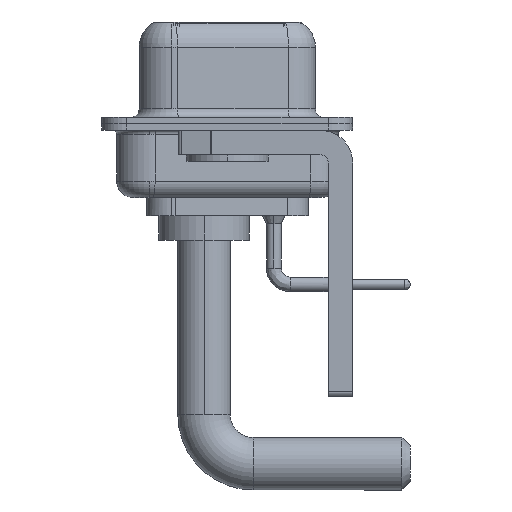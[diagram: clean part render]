
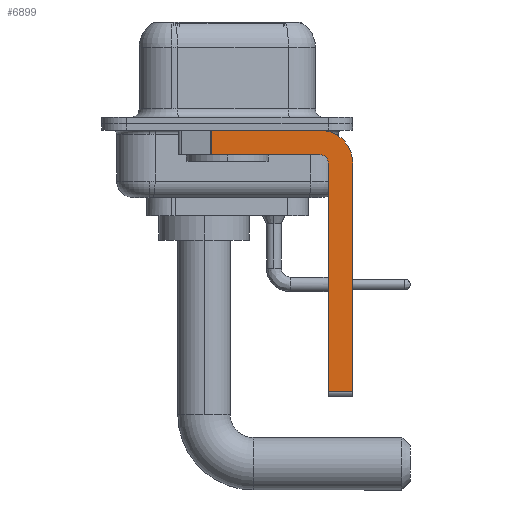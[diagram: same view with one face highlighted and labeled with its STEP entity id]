
A CAD part, left-side view. The second image highlights one B-rep face of the part: STEP entity #6899.
In plain terms, the highlighted planar face has unit normal (-1, 0, 0).
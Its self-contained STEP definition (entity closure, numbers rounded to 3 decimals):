
#76 = VERTEX_POINT ( 'NONE', #11572 ) ;
#138 = AXIS2_PLACEMENT_3D ( 'NONE', #9289, #16056, #19088 ) ;
#366 = CARTESIAN_POINT ( 'NONE',  ( -2.9, -5.65, -0.4 ) ) ;
#731 = LINE ( 'NONE', #9382, #17264 ) ;
#1268 = PLANE ( 'NONE',  #7855 ) ;
#1321 = EDGE_CURVE ( 'NONE', #5923, #15533, #731, .T. ) ;
#2050 = LINE ( 'NONE', #2499, #5967 ) ;
#2391 = ORIENTED_EDGE ( 'NONE', *, *, #16964, .T. ) ;
#2499 = CARTESIAN_POINT ( 'NONE',  ( -2.9, -6.15, -16.6 ) ) ;
#3042 = EDGE_CURVE ( 'NONE', #18371, #21373, #4157, .T. ) ;
#4157 = LINE ( 'NONE', #4265, #19588 ) ;
#4265 = CARTESIAN_POINT ( 'NONE',  ( -2.9, -7.65, -2.4 ) ) ;
#4756 = EDGE_CURVE ( 'NONE', #5923, #18824, #6898, .T. ) ;
#4825 = DIRECTION ( 'NONE',  ( 1., 0., 0. ) ) ;
#4875 = CARTESIAN_POINT ( 'NONE',  ( -2.9, 0.978, -1.9 ) ) ;
#4929 = DIRECTION ( 'NONE',  ( 0., 0., -1. ) ) ;
#5456 = DIRECTION ( 'NONE',  ( 0., 0., -1. ) ) ;
#5864 = DIRECTION ( 'NONE',  ( 0., 1., 0. ) ) ;
#5882 = ORIENTED_EDGE ( 'NONE', *, *, #3042, .F. ) ;
#5923 = VERTEX_POINT ( 'NONE', #16340 ) ;
#5967 = VECTOR ( 'NONE', #12686, 1000. ) ;
#6898 = LINE ( 'NONE', #15528, #19167 ) ;
#6899 = ADVANCED_FACE ( 'NONE', ( #20149 ), #1268, .F. ) ;
#7855 = AXIS2_PLACEMENT_3D ( 'NONE', #11371, #4825, #4929 ) ;
#8131 = LINE ( 'NONE', #14665, #20498 ) ;
#9176 = LINE ( 'NONE', #19524, #13610 ) ;
#9289 = CARTESIAN_POINT ( 'NONE',  ( -2.9, -5.65, -2.4 ) ) ;
#9382 = CARTESIAN_POINT ( 'NONE',  ( -2.9, 3., -0.4 ) ) ;
#9479 = EDGE_CURVE ( 'NONE', #16533, #18824, #9176, .T. ) ;
#9502 = DIRECTION ( 'NONE',  ( 1., 0., 0. ) ) ;
#9514 = EDGE_CURVE ( 'NONE', #76, #16533, #16093, .T. ) ;
#11001 = CIRCLE ( 'NONE', #21680, 2. ) ;
#11037 = DIRECTION ( 'NONE',  ( 0., 0., -1. ) ) ;
#11081 = ORIENTED_EDGE ( 'NONE', *, *, #4756, .T. ) ;
#11094 = ORIENTED_EDGE ( 'NONE', *, *, #20443, .F. ) ;
#11371 = CARTESIAN_POINT ( 'NONE',  ( -2.9, -5.65, -2.4 ) ) ;
#11572 = CARTESIAN_POINT ( 'NONE',  ( -2.9, -6.15, -2.4 ) ) ;
#12342 = CARTESIAN_POINT ( 'NONE',  ( -2.9, -7.65, -16.35 ) ) ;
#12686 = DIRECTION ( 'NONE',  ( 0., 0., 1. ) ) ;
#13154 = CARTESIAN_POINT ( 'NONE',  ( -2.9, -5.65, -2.4 ) ) ;
#13550 = EDGE_LOOP ( 'NONE', ( #18828, #11081, #18710, #16418, #14824, #2391, #5882, #11094 ) ) ;
#13610 = VECTOR ( 'NONE', #5864, 1000. ) ;
#14665 = CARTESIAN_POINT ( 'NONE',  ( -2.9, -5.65, -16.35 ) ) ;
#14824 = ORIENTED_EDGE ( 'NONE', *, *, #16931, .F. ) ;
#15528 = CARTESIAN_POINT ( 'NONE',  ( -2.9, 0.978, -1.9 ) ) ;
#15533 = VERTEX_POINT ( 'NONE', #366 ) ;
#16039 = VERTEX_POINT ( 'NONE', #16734 ) ;
#16056 = DIRECTION ( 'NONE',  ( -1., 0., 0. ) ) ;
#16093 = CIRCLE ( 'NONE', #138, 0.5 ) ;
#16143 = DIRECTION ( 'NONE',  ( 0., -1., 0. ) ) ;
#16340 = CARTESIAN_POINT ( 'NONE',  ( -2.9, 0.978, -0.4 ) ) ;
#16418 = ORIENTED_EDGE ( 'NONE', *, *, #9514, .F. ) ;
#16533 = VERTEX_POINT ( 'NONE', #19838 ) ;
#16734 = CARTESIAN_POINT ( 'NONE',  ( -2.9, -6.15, -16.35 ) ) ;
#16931 = EDGE_CURVE ( 'NONE', #16039, #76, #2050, .T. ) ;
#16964 = EDGE_CURVE ( 'NONE', #16039, #21373, #8131, .T. ) ;
#17264 = VECTOR ( 'NONE', #16143, 1000. ) ;
#17913 = DIRECTION ( 'NONE',  ( 0., -1., 0. ) ) ;
#18371 = VERTEX_POINT ( 'NONE', #18772 ) ;
#18710 = ORIENTED_EDGE ( 'NONE', *, *, #9479, .F. ) ;
#18772 = CARTESIAN_POINT ( 'NONE',  ( -2.9, -7.65, -2.4 ) ) ;
#18824 = VERTEX_POINT ( 'NONE', #4875 ) ;
#18828 = ORIENTED_EDGE ( 'NONE', *, *, #1321, .F. ) ;
#19088 = DIRECTION ( 'NONE',  ( 0., 0., 1. ) ) ;
#19167 = VECTOR ( 'NONE', #5456, 1000. ) ;
#19524 = CARTESIAN_POINT ( 'NONE',  ( -2.9, -5.65, -1.9 ) ) ;
#19588 = VECTOR ( 'NONE', #11037, 1000. ) ;
#19738 = DIRECTION ( 'NONE',  ( 0., 0., -1. ) ) ;
#19838 = CARTESIAN_POINT ( 'NONE',  ( -2.9, -5.65, -1.9 ) ) ;
#20149 = FACE_OUTER_BOUND ( 'NONE', #13550, .T. ) ;
#20443 = EDGE_CURVE ( 'NONE', #15533, #18371, #11001, .T. ) ;
#20498 = VECTOR ( 'NONE', #17913, 1000. ) ;
#21373 = VERTEX_POINT ( 'NONE', #12342 ) ;
#21680 = AXIS2_PLACEMENT_3D ( 'NONE', #13154, #9502, #19738 ) ;
